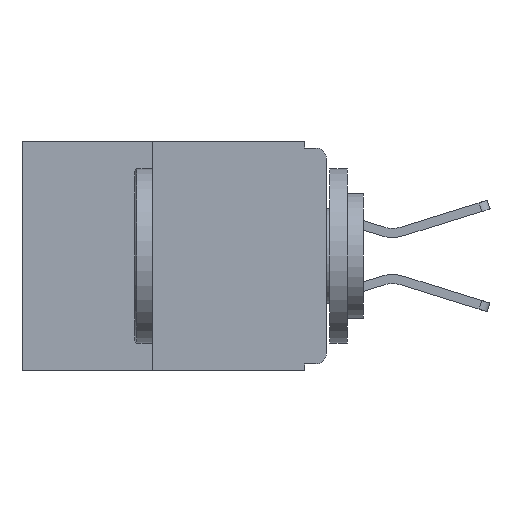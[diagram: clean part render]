
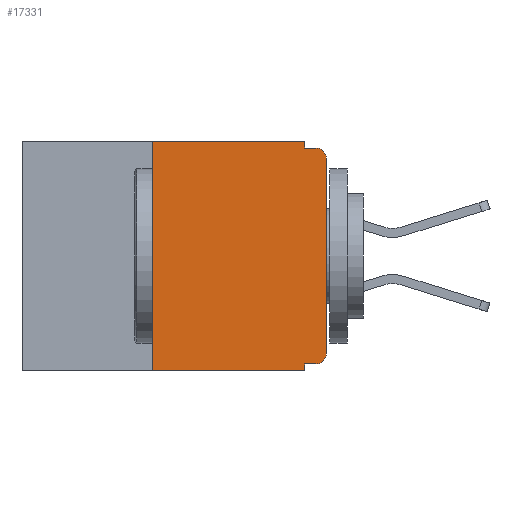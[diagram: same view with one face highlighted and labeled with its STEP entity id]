
A CAD part, left-side view. The second image highlights one B-rep face of the part: STEP entity #17331.
In plain terms, the highlighted planar face has unit normal (-1, 0, 0).
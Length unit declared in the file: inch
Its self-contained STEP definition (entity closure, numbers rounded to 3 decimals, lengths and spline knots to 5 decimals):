
#226 = CARTESIAN_POINT ( 'NONE',  ( 0., 0., -0.01 ) ) ;
#378 = ORIENTED_EDGE ( 'NONE', *, *, #19975, .F. ) ;
#724 = VECTOR ( 'NONE', #24453, 39.37008 ) ;
#761 = AXIS2_PLACEMENT_3D ( 'NONE', #8475, #22020, #10464 ) ;
#787 = DIRECTION ( 'NONE',  ( 0., -1., 0. ) ) ;
#924 = VERTEX_POINT ( 'NONE', #24233 ) ;
#1258 = CARTESIAN_POINT ( 'NONE',  ( 0., 0.25, -0.33 ) ) ;
#1289 = ORIENTED_EDGE ( 'NONE', *, *, #4348, .T. ) ;
#1705 = DIRECTION ( 'NONE',  ( 0., -1., 0. ) ) ;
#1833 = LINE ( 'NONE', #19717, #17402 ) ;
#2894 = FACE_OUTER_BOUND ( 'NONE', #24854, .T. ) ;
#3086 = CARTESIAN_POINT ( 'NONE',  ( 0., 0., -0.305 ) ) ;
#3231 = DIRECTION ( 'NONE',  ( 0., 0., 1. ) ) ;
#3406 = VERTEX_POINT ( 'NONE', #23785 ) ;
#4348 = EDGE_CURVE ( 'NONE', #14211, #9566, #1833, .T. ) ;
#5056 = DIRECTION ( 'NONE',  ( 0., 0., -1. ) ) ;
#5567 = CARTESIAN_POINT ( 'NONE',  ( 0., 0.437, 0. ) ) ;
#5881 = LINE ( 'NONE', #226, #20769 ) ;
#6226 = ORIENTED_EDGE ( 'NONE', *, *, #9511, .T. ) ;
#6516 = ORIENTED_EDGE ( 'NONE', *, *, #13372, .T. ) ;
#6519 = LINE ( 'NONE', #20789, #12963 ) ;
#6838 = VERTEX_POINT ( 'NONE', #9980 ) ;
#6993 = EDGE_CURVE ( 'NONE', #21582, #924, #11210, .T. ) ;
#7534 = DIRECTION ( 'NONE',  ( 1., 0., 0. ) ) ;
#7873 = EDGE_CURVE ( 'NONE', #6838, #8741, #6519, .T. ) ;
#8475 = CARTESIAN_POINT ( 'NONE',  ( 0., 0.015, -0.025 ) ) ;
#8530 = VERTEX_POINT ( 'NONE', #24911 ) ;
#8741 = VERTEX_POINT ( 'NONE', #22807 ) ;
#9039 = VERTEX_POINT ( 'NONE', #18962 ) ;
#9511 = EDGE_CURVE ( 'NONE', #9039, #14211, #13965, .T. ) ;
#9566 = VERTEX_POINT ( 'NONE', #13230 ) ;
#9582 = DIRECTION ( 'NONE',  ( 0., 1., 0. ) ) ;
#9980 = CARTESIAN_POINT ( 'NONE',  ( 0., 0.25, -0.33 ) ) ;
#10085 = AXIS2_PLACEMENT_3D ( 'NONE', #5567, #7534, #21134 ) ;
#10464 = DIRECTION ( 'NONE',  ( 0., 0., -1. ) ) ;
#11210 = LINE ( 'NONE', #22160, #724 ) ;
#11395 = LINE ( 'NONE', #1258, #21057 ) ;
#11543 = CARTESIAN_POINT ( 'NONE',  ( 0., 0., -0.32 ) ) ;
#11602 = EDGE_CURVE ( 'NONE', #924, #8530, #5881, .T. ) ;
#11817 = LINE ( 'NONE', #20609, #16947 ) ;
#12262 = VERTEX_POINT ( 'NONE', #16770 ) ;
#12700 = VECTOR ( 'NONE', #1705, 39.37008 ) ;
#12914 = EDGE_CURVE ( 'NONE', #6838, #3406, #11395, .T. ) ;
#12963 = VECTOR ( 'NONE', #20427, 39.37008 ) ;
#13230 = CARTESIAN_POINT ( 'NONE',  ( 0., 0., -0.025 ) ) ;
#13311 = LINE ( 'NONE', #24892, #12700 ) ;
#13372 = EDGE_CURVE ( 'NONE', #9566, #8530, #15891, .T. ) ;
#13524 = DIRECTION ( 'NONE',  ( 0., 0., -1. ) ) ;
#13582 = DIRECTION ( 'NONE',  ( -1., 0., 0. ) ) ;
#13589 = CARTESIAN_POINT ( 'NONE',  ( 0., 0.015, -0.305 ) ) ;
#13965 = CIRCLE ( 'NONE', #18034, 0.015 ) ;
#14211 = VERTEX_POINT ( 'NONE', #3086 ) ;
#14610 = CARTESIAN_POINT ( 'NONE',  ( 0., 0.031, 0. ) ) ;
#15891 = CIRCLE ( 'NONE', #761, 0.015 ) ;
#16770 = CARTESIAN_POINT ( 'NONE',  ( 0., 0.031, -0.32 ) ) ;
#16947 = VECTOR ( 'NONE', #5056, 39.37008 ) ;
#17182 = EDGE_CURVE ( 'NONE', #12262, #8741, #11817, .T. ) ;
#17331 = ADVANCED_FACE ( 'NONE', ( #2894 ), #24816, .F. ) ;
#17340 = EDGE_CURVE ( 'NONE', #3406, #21582, #13311, .T. ) ;
#17402 = VECTOR ( 'NONE', #18968, 39.37008 ) ;
#18034 = AXIS2_PLACEMENT_3D ( 'NONE', #13589, #13582, #13524 ) ;
#18095 = ORIENTED_EDGE ( 'NONE', *, *, #11602, .F. ) ;
#18962 = CARTESIAN_POINT ( 'NONE',  ( 0., 0.015, -0.32 ) ) ;
#18968 = DIRECTION ( 'NONE',  ( 0., 0., 1. ) ) ;
#19249 = VECTOR ( 'NONE', #9582, 39.37008 ) ;
#19317 = ORIENTED_EDGE ( 'NONE', *, *, #6993, .F. ) ;
#19717 = CARTESIAN_POINT ( 'NONE',  ( 0., 0., 0. ) ) ;
#19866 = LINE ( 'NONE', #11543, #19249 ) ;
#19932 = ORIENTED_EDGE ( 'NONE', *, *, #12914, .F. ) ;
#19975 = EDGE_CURVE ( 'NONE', #9039, #12262, #19866, .T. ) ;
#20427 = DIRECTION ( 'NONE',  ( 0., -1., 0. ) ) ;
#20507 = ORIENTED_EDGE ( 'NONE', *, *, #17182, .F. ) ;
#20609 = CARTESIAN_POINT ( 'NONE',  ( 0., 0.031, -0.33 ) ) ;
#20769 = VECTOR ( 'NONE', #787, 39.37008 ) ;
#20789 = CARTESIAN_POINT ( 'NONE',  ( 0., 0.437, -0.33 ) ) ;
#21057 = VECTOR ( 'NONE', #3231, 39.37008 ) ;
#21134 = DIRECTION ( 'NONE',  ( 0., 0., -1. ) ) ;
#21582 = VERTEX_POINT ( 'NONE', #14610 ) ;
#22020 = DIRECTION ( 'NONE',  ( -1., 0., 0. ) ) ;
#22160 = CARTESIAN_POINT ( 'NONE',  ( 0., 0.031, 0. ) ) ;
#22807 = CARTESIAN_POINT ( 'NONE',  ( 0., 0.031, -0.33 ) ) ;
#23785 = CARTESIAN_POINT ( 'NONE',  ( 0., 0.25, 0. ) ) ;
#24233 = CARTESIAN_POINT ( 'NONE',  ( 0., 0.031, -0.01 ) ) ;
#24354 = ORIENTED_EDGE ( 'NONE', *, *, #17340, .F. ) ;
#24453 = DIRECTION ( 'NONE',  ( 0., 0., -1. ) ) ;
#24816 = PLANE ( 'NONE',  #10085 ) ;
#24854 = EDGE_LOOP ( 'NONE', ( #1289, #6516, #18095, #19317, #24354, #19932, #24948, #20507, #378, #6226 ) ) ;
#24892 = CARTESIAN_POINT ( 'NONE',  ( 0., 0.437, 0. ) ) ;
#24911 = CARTESIAN_POINT ( 'NONE',  ( 0., 0.015, -0.01 ) ) ;
#24948 = ORIENTED_EDGE ( 'NONE', *, *, #7873, .T. ) ;
